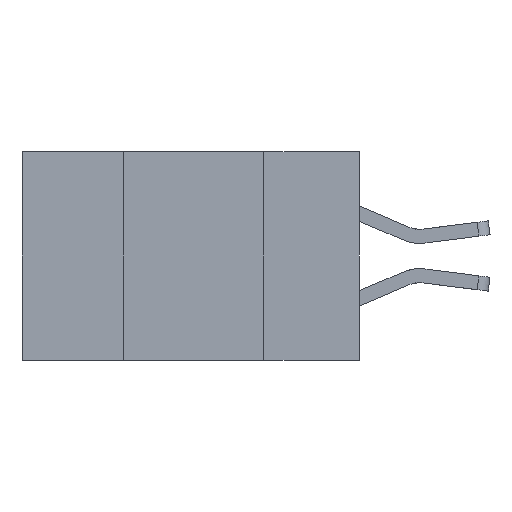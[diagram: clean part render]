
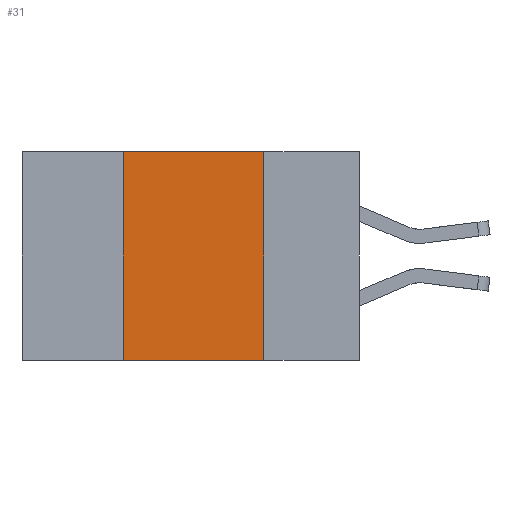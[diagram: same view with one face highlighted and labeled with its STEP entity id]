
A CAD part, left-side view. The second image highlights one B-rep face of the part: STEP entity #31.
In plain terms, the highlighted planar face has unit normal (-1, 0, 0).
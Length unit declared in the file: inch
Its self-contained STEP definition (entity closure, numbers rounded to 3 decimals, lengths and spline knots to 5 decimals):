
#31 = ADVANCED_FACE ( 'NONE', ( #6951 ), #3926, .F. ) ;
#135 = VECTOR ( 'NONE', #4467, 39.37008 ) ;
#407 = VECTOR ( 'NONE', #4586, 39.37008 ) ;
#682 = DIRECTION ( 'NONE',  ( 0., -1., 0. ) ) ;
#1194 = VERTEX_POINT ( 'NONE', #8056 ) ;
#1577 = CARTESIAN_POINT ( 'NONE',  ( 0., 0.42, -0.37 ) ) ;
#1736 = VERTEX_POINT ( 'NONE', #7462 ) ;
#2249 = LINE ( 'NONE', #8801, #6626 ) ;
#2674 = DIRECTION ( 'NONE',  ( 0., 0., -1. ) ) ;
#2959 = LINE ( 'NONE', #11141, #7290 ) ;
#3127 = VERTEX_POINT ( 'NONE', #4843 ) ;
#3634 = DIRECTION ( 'NONE',  ( 0., 0., 1. ) ) ;
#3866 = EDGE_LOOP ( 'NONE', ( #5619, #3916, #5017, #9043 ) ) ;
#3916 = ORIENTED_EDGE ( 'NONE', *, *, #5423, .F. ) ;
#3926 = PLANE ( 'NONE',  #7009 ) ;
#4467 = DIRECTION ( 'NONE',  ( 0., 0., -1. ) ) ;
#4492 = CARTESIAN_POINT ( 'NONE',  ( 0., 0.17, 0. ) ) ;
#4586 = DIRECTION ( 'NONE',  ( 0., -1., 0. ) ) ;
#4614 = CARTESIAN_POINT ( 'NONE',  ( 0., 0.6, 0. ) ) ;
#4843 = CARTESIAN_POINT ( 'NONE',  ( 0., 0.17, -0.37 ) ) ;
#4944 = LINE ( 'NONE', #4492, #135 ) ;
#5017 = ORIENTED_EDGE ( 'NONE', *, *, #6568, .F. ) ;
#5423 = EDGE_CURVE ( 'NONE', #1194, #1736, #5476, .T. ) ;
#5453 = EDGE_CURVE ( 'NONE', #1736, #3127, #4944, .T. ) ;
#5476 = LINE ( 'NONE', #4614, #407 ) ;
#5619 = ORIENTED_EDGE ( 'NONE', *, *, #5453, .F. ) ;
#5947 = VERTEX_POINT ( 'NONE', #1577 ) ;
#6568 = EDGE_CURVE ( 'NONE', #5947, #1194, #2249, .T. ) ;
#6626 = VECTOR ( 'NONE', #3634, 39.37008 ) ;
#6951 = FACE_OUTER_BOUND ( 'NONE', #3866, .T. ) ;
#7009 = AXIS2_PLACEMENT_3D ( 'NONE', #10384, #7881, #2674 ) ;
#7290 = VECTOR ( 'NONE', #682, 39.37008 ) ;
#7462 = CARTESIAN_POINT ( 'NONE',  ( 0., 0.17, 0. ) ) ;
#7881 = DIRECTION ( 'NONE',  ( 1., 0., 0. ) ) ;
#8056 = CARTESIAN_POINT ( 'NONE',  ( 0., 0.42, 0. ) ) ;
#8801 = CARTESIAN_POINT ( 'NONE',  ( 0., 0.42, 0. ) ) ;
#9043 = ORIENTED_EDGE ( 'NONE', *, *, #10279, .T. ) ;
#10279 = EDGE_CURVE ( 'NONE', #5947, #3127, #2959, .T. ) ;
#10384 = CARTESIAN_POINT ( 'NONE',  ( 0., 0.6, 0. ) ) ;
#11141 = CARTESIAN_POINT ( 'NONE',  ( 0., 0.6, -0.37 ) ) ;
